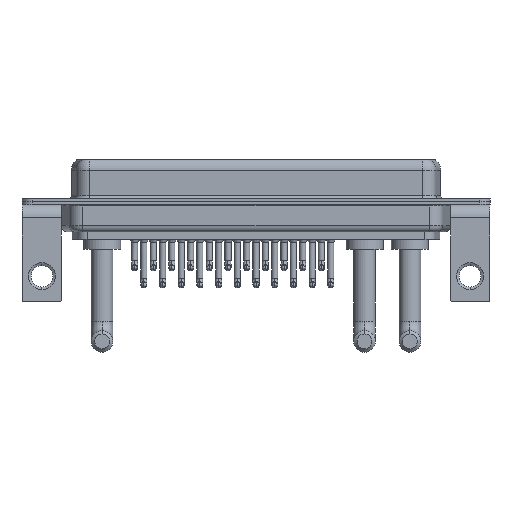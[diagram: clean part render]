
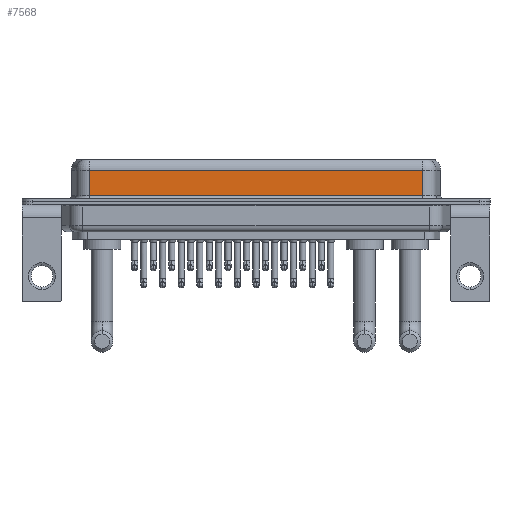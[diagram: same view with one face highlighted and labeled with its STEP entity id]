
A CAD part, front view. The second image highlights one B-rep face of the part: STEP entity #7568.
In plain terms, the highlighted planar face has unit normal (0, -1, 0).
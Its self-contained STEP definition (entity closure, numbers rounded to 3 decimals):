
#179 = CARTESIAN_POINT ( 'NONE',  ( 56.462, -3.95, 4.65 ) ) ;
#672 = CARTESIAN_POINT ( 'NONE',  ( 7.038, -3.95, 4.65 ) ) ;
#1249 = ORIENTED_EDGE ( 'NONE', *, *, #20204, .T. ) ;
#1295 = CARTESIAN_POINT ( 'NONE',  ( 56.462, -3.95, 0.9 ) ) ;
#3157 = CARTESIAN_POINT ( 'NONE',  ( 56.462, -3.95, 0.9 ) ) ;
#3581 = VECTOR ( 'NONE', #22423, 1000. ) ;
#3807 = VECTOR ( 'NONE', #19944, 1000. ) ;
#4169 = DIRECTION ( 'NONE',  ( 0., 0., -1. ) ) ;
#4209 = VERTEX_POINT ( 'NONE', #672 ) ;
#4398 = VERTEX_POINT ( 'NONE', #3157 ) ;
#4757 = EDGE_CURVE ( 'NONE', #4209, #20605, #23136, .T. ) ;
#6283 = DIRECTION ( 'NONE',  ( 0., 1., 0. ) ) ;
#7007 = ORIENTED_EDGE ( 'NONE', *, *, #4757, .T. ) ;
#7355 = EDGE_CURVE ( 'NONE', #20605, #4398, #21816, .T. ) ;
#7537 = EDGE_CURVE ( 'NONE', #16048, #4398, #15819, .T. ) ;
#7568 = ADVANCED_FACE ( 'NONE', ( #17442 ), #12114, .F. ) ;
#9122 = CARTESIAN_POINT ( 'NONE',  ( 7.038, -3.95, 0.9 ) ) ;
#11023 = CARTESIAN_POINT ( 'NONE',  ( 56.462, -3.95, 4.65 ) ) ;
#12114 = PLANE ( 'NONE',  #13759 ) ;
#13459 = DIRECTION ( 'NONE',  ( 0., 0., -1. ) ) ;
#13759 = AXIS2_PLACEMENT_3D ( 'NONE', #23259, #6283, #19297 ) ;
#14858 = LINE ( 'NONE', #11023, #3581 ) ;
#15270 = EDGE_LOOP ( 'NONE', ( #19251, #1249, #7007, #20729 ) ) ;
#15819 = LINE ( 'NONE', #21301, #19293 ) ;
#16048 = VERTEX_POINT ( 'NONE', #179 ) ;
#17442 = FACE_OUTER_BOUND ( 'NONE', #15270, .T. ) ;
#17873 = VECTOR ( 'NONE', #13459, 1000. ) ;
#19251 = ORIENTED_EDGE ( 'NONE', *, *, #7537, .F. ) ;
#19293 = VECTOR ( 'NONE', #4169, 1000. ) ;
#19297 = DIRECTION ( 'NONE',  ( 0., 0., 1. ) ) ;
#19944 = DIRECTION ( 'NONE',  ( 1., 0., 0. ) ) ;
#20204 = EDGE_CURVE ( 'NONE', #16048, #4209, #14858, .T. ) ;
#20605 = VERTEX_POINT ( 'NONE', #9122 ) ;
#20729 = ORIENTED_EDGE ( 'NONE', *, *, #7355, .T. ) ;
#21167 = CARTESIAN_POINT ( 'NONE',  ( 7.038, -3.95, 6.4 ) ) ;
#21301 = CARTESIAN_POINT ( 'NONE',  ( 56.462, -3.95, 6.4 ) ) ;
#21816 = LINE ( 'NONE', #1295, #3807 ) ;
#22423 = DIRECTION ( 'NONE',  ( -1., 0., 0. ) ) ;
#23136 = LINE ( 'NONE', #21167, #17873 ) ;
#23259 = CARTESIAN_POINT ( 'NONE',  ( 56.462, -3.95, 6.4 ) ) ;
